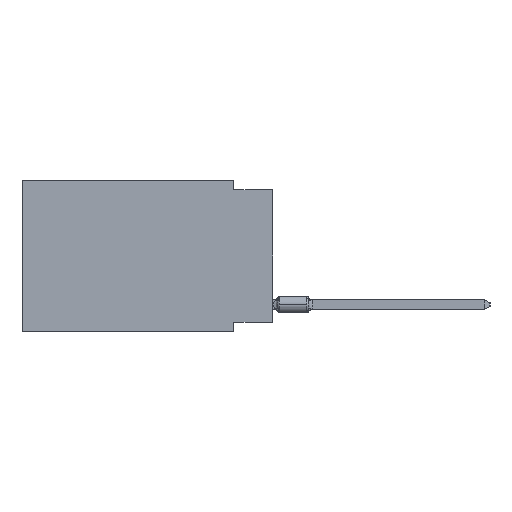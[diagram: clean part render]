
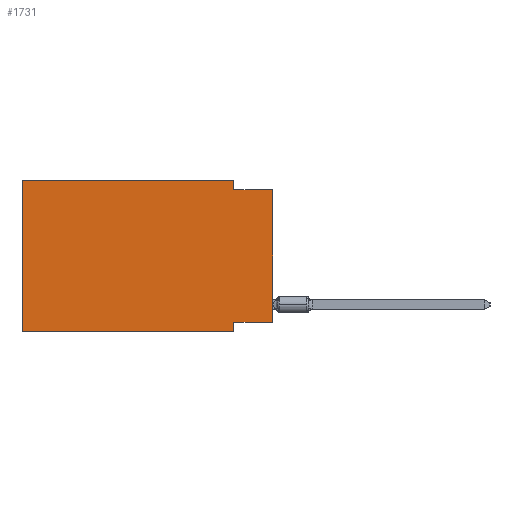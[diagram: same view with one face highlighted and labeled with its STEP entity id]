
A CAD part, left-side view. The second image highlights one B-rep face of the part: STEP entity #1731.
In plain terms, the highlighted planar face has unit normal (-1, 0, 0).
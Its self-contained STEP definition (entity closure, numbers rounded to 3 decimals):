
#405 = DIRECTION ( 'NONE',  ( 0., -1., 0. ) ) ;
#760 = VERTEX_POINT ( 'NONE', #31481 ) ;
#1269 = VERTEX_POINT ( 'NONE', #35602 ) ;
#1731 = ADVANCED_FACE ( 'NONE', ( #3098 ), #8383, .F. ) ;
#1858 = VERTEX_POINT ( 'NONE', #10372 ) ;
#2394 = ORIENTED_EDGE ( 'NONE', *, *, #12762, .F. ) ;
#2547 = CARTESIAN_POINT ( 'NONE',  ( 0., 16.383, 0. ) ) ;
#3098 = FACE_OUTER_BOUND ( 'NONE', #5183, .T. ) ;
#3101 = ORIENTED_EDGE ( 'NONE', *, *, #13688, .F. ) ;
#3396 = LINE ( 'NONE', #11957, #5389 ) ;
#3449 = ORIENTED_EDGE ( 'NONE', *, *, #31478, .F. ) ;
#3462 = DIRECTION ( 'NONE',  ( 0., 1., 0. ) ) ;
#3501 = LINE ( 'NONE', #26299, #22199 ) ;
#3903 = CARTESIAN_POINT ( 'NONE',  ( 0., 0., -0.635 ) ) ;
#3997 = CARTESIAN_POINT ( 'NONE',  ( 0., 2.54, -0.635 ) ) ;
#5112 = DIRECTION ( 'NONE',  ( 0., -1., 0. ) ) ;
#5183 = EDGE_LOOP ( 'NONE', ( #7760, #31250, #19918, #21580, #2394, #16948, #3101, #3449 ) ) ;
#5389 = VECTOR ( 'NONE', #31135, 1000. ) ;
#6233 = DIRECTION ( 'NONE',  ( 0., 0., -1. ) ) ;
#7675 = CARTESIAN_POINT ( 'NONE',  ( 0., 16.383, 0. ) ) ;
#7760 = ORIENTED_EDGE ( 'NONE', *, *, #27321, .T. ) ;
#8181 = VERTEX_POINT ( 'NONE', #3903 ) ;
#8285 = EDGE_CURVE ( 'NONE', #23177, #1269, #29281, .T. ) ;
#8383 = PLANE ( 'NONE',  #10016 ) ;
#8560 = DIRECTION ( 'NONE',  ( 0., 0., -1. ) ) ;
#8600 = VERTEX_POINT ( 'NONE', #3997 ) ;
#9892 = CARTESIAN_POINT ( 'NONE',  ( 0., 0., 0. ) ) ;
#10016 = AXIS2_PLACEMENT_3D ( 'NONE', #2547, #30277, #8560 ) ;
#10372 = CARTESIAN_POINT ( 'NONE',  ( 0., 2.54, -9.906 ) ) ;
#10616 = VERTEX_POINT ( 'NONE', #12485 ) ;
#11320 = LINE ( 'NONE', #19348, #12116 ) ;
#11957 = CARTESIAN_POINT ( 'NONE',  ( 0., 2.54, 0. ) ) ;
#12116 = VECTOR ( 'NONE', #22449, 1000. ) ;
#12485 = CARTESIAN_POINT ( 'NONE',  ( 0., 0., -9.271 ) ) ;
#12762 = EDGE_CURVE ( 'NONE', #29305, #23177, #11320, .T. ) ;
#13688 = EDGE_CURVE ( 'NONE', #760, #1858, #3501, .T. ) ;
#14273 = LINE ( 'NONE', #25400, #26069 ) ;
#14766 = CARTESIAN_POINT ( 'NONE',  ( 0., 0., -9.271 ) ) ;
#16948 = ORIENTED_EDGE ( 'NONE', *, *, #19404, .T. ) ;
#18032 = CARTESIAN_POINT ( 'NONE',  ( 0., 16.383, 0. ) ) ;
#18604 = LINE ( 'NONE', #29748, #31241 ) ;
#19348 = CARTESIAN_POINT ( 'NONE',  ( 0., 16.383, 0. ) ) ;
#19404 = EDGE_CURVE ( 'NONE', #29305, #1858, #18604, .T. ) ;
#19918 = ORIENTED_EDGE ( 'NONE', *, *, #28432, .F. ) ;
#20476 = VECTOR ( 'NONE', #26853, 1000. ) ;
#21148 = VECTOR ( 'NONE', #5112, 1000. ) ;
#21190 = LINE ( 'NONE', #9892, #20476 ) ;
#21580 = ORIENTED_EDGE ( 'NONE', *, *, #8285, .F. ) ;
#22199 = VECTOR ( 'NONE', #6233, 1000. ) ;
#22292 = EDGE_CURVE ( 'NONE', #8600, #8181, #14273, .T. ) ;
#22449 = DIRECTION ( 'NONE',  ( 0., 0., 1. ) ) ;
#23177 = VERTEX_POINT ( 'NONE', #18032 ) ;
#23496 = CARTESIAN_POINT ( 'NONE',  ( 0., 16.383, -9.906 ) ) ;
#24894 = VECTOR ( 'NONE', #3462, 1000. ) ;
#25400 = CARTESIAN_POINT ( 'NONE',  ( 0., 0., -0.635 ) ) ;
#26069 = VECTOR ( 'NONE', #405, 1000. ) ;
#26071 = LINE ( 'NONE', #14766, #24894 ) ;
#26299 = CARTESIAN_POINT ( 'NONE',  ( 0., 2.54, -9.906 ) ) ;
#26473 = DIRECTION ( 'NONE',  ( 0., -1., 0. ) ) ;
#26853 = DIRECTION ( 'NONE',  ( 0., 0., 1. ) ) ;
#27321 = EDGE_CURVE ( 'NONE', #10616, #8181, #21190, .T. ) ;
#28432 = EDGE_CURVE ( 'NONE', #1269, #8600, #3396, .T. ) ;
#29281 = LINE ( 'NONE', #7675, #21148 ) ;
#29305 = VERTEX_POINT ( 'NONE', #23496 ) ;
#29748 = CARTESIAN_POINT ( 'NONE',  ( 0., 16.383, -9.906 ) ) ;
#30277 = DIRECTION ( 'NONE',  ( 1., 0., 0. ) ) ;
#31135 = DIRECTION ( 'NONE',  ( 0., 0., -1. ) ) ;
#31241 = VECTOR ( 'NONE', #26473, 1000. ) ;
#31250 = ORIENTED_EDGE ( 'NONE', *, *, #22292, .F. ) ;
#31478 = EDGE_CURVE ( 'NONE', #10616, #760, #26071, .T. ) ;
#31481 = CARTESIAN_POINT ( 'NONE',  ( 0., 2.54, -9.271 ) ) ;
#35602 = CARTESIAN_POINT ( 'NONE',  ( 0., 2.54, 0. ) ) ;
